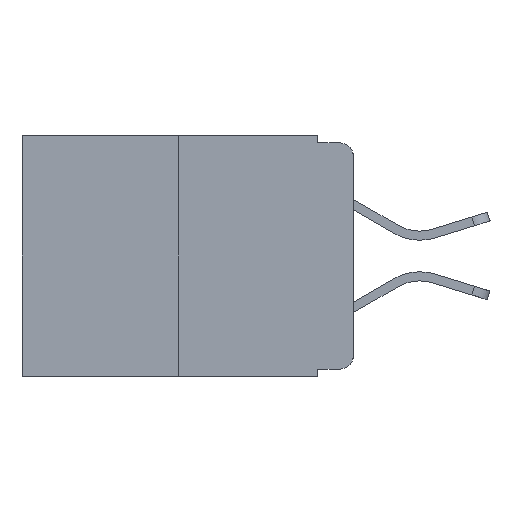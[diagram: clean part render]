
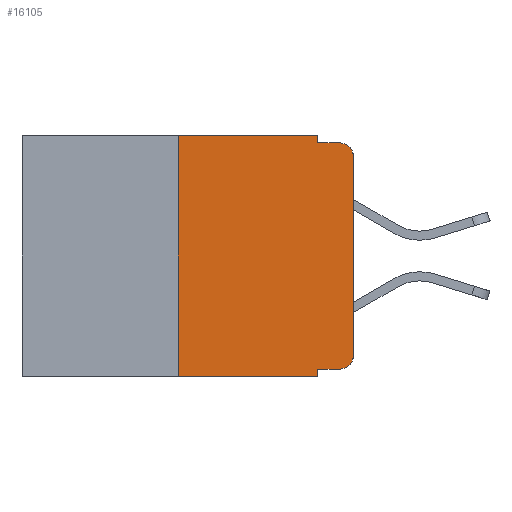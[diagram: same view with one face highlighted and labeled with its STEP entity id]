
A CAD part, left-side view. The second image highlights one B-rep face of the part: STEP entity #16105.
In plain terms, the highlighted planar face has unit normal (-1, 0, 0).
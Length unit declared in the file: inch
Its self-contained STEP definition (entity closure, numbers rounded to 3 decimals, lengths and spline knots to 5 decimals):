
#404 = VECTOR ( 'NONE', #16312, 39.37008 ) ;
#654 = EDGE_CURVE ( 'NONE', #7976, #4614, #12950, .T. ) ;
#694 = ORIENTED_EDGE ( 'NONE', *, *, #1496, .F. ) ;
#701 = DIRECTION ( 'NONE',  ( 0., 0., -1. ) ) ;
#882 = EDGE_CURVE ( 'NONE', #5076, #6042, #3626, .T. ) ;
#994 = ORIENTED_EDGE ( 'NONE', *, *, #10132, .F. ) ;
#1006 = DIRECTION ( 'NONE',  ( 0., 0., 1. ) ) ;
#1008 = AXIS2_PLACEMENT_3D ( 'NONE', #7092, #12230, #8260 ) ;
#1496 = EDGE_CURVE ( 'NONE', #8031, #3222, #10059, .T. ) ;
#1594 = CARTESIAN_POINT ( 'NONE',  ( 0., 0.051, 0. ) ) ;
#2262 = DIRECTION ( 'NONE',  ( 0., -1., 0. ) ) ;
#2353 = AXIS2_PLACEMENT_3D ( 'NONE', #13265, #6895, #7702 ) ;
#2384 = VECTOR ( 'NONE', #701, 39.37008 ) ;
#2466 = DIRECTION ( 'NONE',  ( 1., 0., 0. ) ) ;
#2535 = VECTOR ( 'NONE', #10715, 39.37008 ) ;
#3222 = VERTEX_POINT ( 'NONE', #13737 ) ;
#3472 = CARTESIAN_POINT ( 'NONE',  ( 0., 0.051, -0.333 ) ) ;
#3498 = ORIENTED_EDGE ( 'NONE', *, *, #7003, .T. ) ;
#3626 = LINE ( 'NONE', #10351, #10492 ) ;
#3693 = CARTESIAN_POINT ( 'NONE',  ( 0., 0.25, 0. ) ) ;
#3723 = EDGE_CURVE ( 'NONE', #12888, #12117, #10389, .T. ) ;
#3883 = FACE_OUTER_BOUND ( 'NONE', #15416, .T. ) ;
#4077 = CARTESIAN_POINT ( 'NONE',  ( 0., 0.473, -0.343 ) ) ;
#4353 = VECTOR ( 'NONE', #12172, 39.37008 ) ;
#4614 = VERTEX_POINT ( 'NONE', #6221 ) ;
#4651 = VECTOR ( 'NONE', #5830, 39.37008 ) ;
#4834 = CARTESIAN_POINT ( 'NONE',  ( 0., 0.051, -0.01 ) ) ;
#5076 = VERTEX_POINT ( 'NONE', #16590 ) ;
#5198 = CARTESIAN_POINT ( 'NONE',  ( 0., 0.25, -0.343 ) ) ;
#5830 = DIRECTION ( 'NONE',  ( 0., -1., 0. ) ) ;
#6042 = VERTEX_POINT ( 'NONE', #12294 ) ;
#6106 = EDGE_CURVE ( 'NONE', #8964, #5076, #9257, .T. ) ;
#6193 = LINE ( 'NONE', #7604, #10352 ) ;
#6221 = CARTESIAN_POINT ( 'NONE',  ( 0., 0.02, -0.01 ) ) ;
#6253 = LINE ( 'NONE', #1594, #2535 ) ;
#6536 = ORIENTED_EDGE ( 'NONE', *, *, #14799, .F. ) ;
#6878 = ORIENTED_EDGE ( 'NONE', *, *, #654, .F. ) ;
#6895 = DIRECTION ( 'NONE',  ( -1., 0., 0. ) ) ;
#7003 = EDGE_CURVE ( 'NONE', #6042, #4614, #13425, .T. ) ;
#7092 = CARTESIAN_POINT ( 'NONE',  ( 0., 0.02, -0.313 ) ) ;
#7255 = CARTESIAN_POINT ( 'NONE',  ( 0., 0.051, 0. ) ) ;
#7604 = CARTESIAN_POINT ( 'NONE',  ( 0., 0.25, 0. ) ) ;
#7702 = DIRECTION ( 'NONE',  ( 0., 0., -1. ) ) ;
#7976 = VERTEX_POINT ( 'NONE', #4834 ) ;
#8031 = VERTEX_POINT ( 'NONE', #16910 ) ;
#8165 = VECTOR ( 'NONE', #2262, 39.37008 ) ;
#8260 = DIRECTION ( 'NONE',  ( 0., 0., -1. ) ) ;
#8618 = CARTESIAN_POINT ( 'NONE',  ( 0., 0.051, -0.01 ) ) ;
#8964 = VERTEX_POINT ( 'NONE', #10859 ) ;
#9192 = EDGE_CURVE ( 'NONE', #8031, #8964, #10676, .T. ) ;
#9257 = CIRCLE ( 'NONE', #1008, 0.02 ) ;
#9639 = CARTESIAN_POINT ( 'NONE',  ( 0., 0.473, 0. ) ) ;
#10059 = LINE ( 'NONE', #7255, #2384 ) ;
#10132 = EDGE_CURVE ( 'NONE', #12117, #7976, #6253, .T. ) ;
#10233 = AXIS2_PLACEMENT_3D ( 'NONE', #10467, #2466, #13120 ) ;
#10351 = CARTESIAN_POINT ( 'NONE',  ( 0., 0., 0. ) ) ;
#10352 = VECTOR ( 'NONE', #1006, 39.37008 ) ;
#10389 = LINE ( 'NONE', #9639, #404 ) ;
#10467 = CARTESIAN_POINT ( 'NONE',  ( 0., 0.473, 0. ) ) ;
#10492 = VECTOR ( 'NONE', #11665, 39.37008 ) ;
#10676 = LINE ( 'NONE', #3472, #8165 ) ;
#10715 = DIRECTION ( 'NONE',  ( 0., 0., -1. ) ) ;
#10797 = ORIENTED_EDGE ( 'NONE', *, *, #6106, .T. ) ;
#10859 = CARTESIAN_POINT ( 'NONE',  ( 0., 0.02, -0.333 ) ) ;
#10866 = ORIENTED_EDGE ( 'NONE', *, *, #9192, .T. ) ;
#11665 = DIRECTION ( 'NONE',  ( 0., 0., 1. ) ) ;
#12117 = VERTEX_POINT ( 'NONE', #12344 ) ;
#12172 = DIRECTION ( 'NONE',  ( 0., -1., 0. ) ) ;
#12230 = DIRECTION ( 'NONE',  ( -1., 0., 0. ) ) ;
#12294 = CARTESIAN_POINT ( 'NONE',  ( 0., 0., -0.03 ) ) ;
#12344 = CARTESIAN_POINT ( 'NONE',  ( 0., 0.051, 0. ) ) ;
#12860 = LINE ( 'NONE', #4077, #4353 ) ;
#12861 = VERTEX_POINT ( 'NONE', #5198 ) ;
#12888 = VERTEX_POINT ( 'NONE', #3693 ) ;
#12950 = LINE ( 'NONE', #8618, #4651 ) ;
#13120 = DIRECTION ( 'NONE',  ( 0., 0., -1. ) ) ;
#13265 = CARTESIAN_POINT ( 'NONE',  ( 0., 0.02, -0.03 ) ) ;
#13425 = CIRCLE ( 'NONE', #2353, 0.02 ) ;
#13737 = CARTESIAN_POINT ( 'NONE',  ( 0., 0.051, -0.343 ) ) ;
#13795 = EDGE_CURVE ( 'NONE', #12861, #3222, #12860, .T. ) ;
#14463 = PLANE ( 'NONE',  #10233 ) ;
#14799 = EDGE_CURVE ( 'NONE', #12861, #12888, #6193, .T. ) ;
#15416 = EDGE_LOOP ( 'NONE', ( #16719, #3498, #6878, #994, #16310, #6536, #16901, #694, #10866, #10797 ) ) ;
#16105 = ADVANCED_FACE ( 'NONE', ( #3883 ), #14463, .F. ) ;
#16310 = ORIENTED_EDGE ( 'NONE', *, *, #3723, .F. ) ;
#16312 = DIRECTION ( 'NONE',  ( 0., -1., 0. ) ) ;
#16590 = CARTESIAN_POINT ( 'NONE',  ( 0., 0., -0.313 ) ) ;
#16719 = ORIENTED_EDGE ( 'NONE', *, *, #882, .T. ) ;
#16901 = ORIENTED_EDGE ( 'NONE', *, *, #13795, .T. ) ;
#16910 = CARTESIAN_POINT ( 'NONE',  ( 0., 0.051, -0.333 ) ) ;
